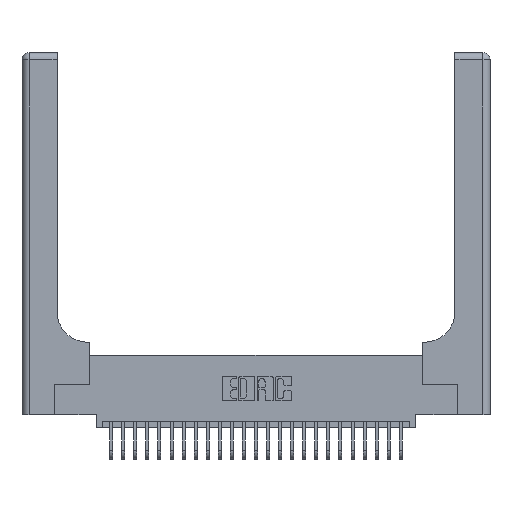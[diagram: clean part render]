
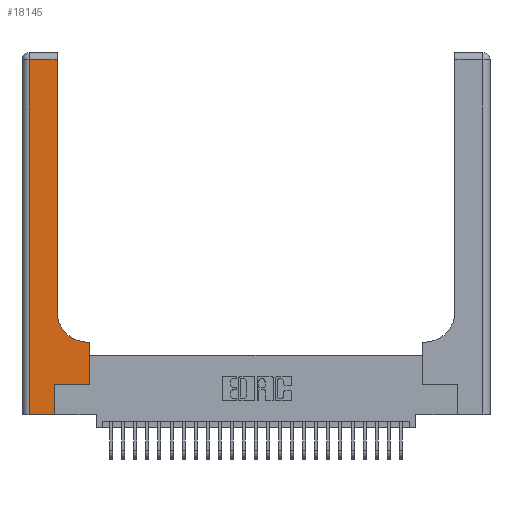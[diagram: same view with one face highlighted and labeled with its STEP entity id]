
A CAD part, top view. The second image highlights one B-rep face of the part: STEP entity #18145.
In plain terms, the highlighted planar face has unit normal (0, 0, 1).
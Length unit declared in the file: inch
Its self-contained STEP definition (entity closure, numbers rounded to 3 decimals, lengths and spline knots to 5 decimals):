
#85 = DIRECTION ( 'NONE',  ( 0., 1., 0. ) ) ;
#137 = CARTESIAN_POINT ( 'NONE',  ( 0.06, 2.94, 0.37 ) ) ;
#306 = VECTOR ( 'NONE', #23178, 39.37008 ) ;
#608 = VERTEX_POINT ( 'NONE', #1869 ) ;
#842 = DIRECTION ( 'NONE',  ( 0., 1., 0. ) ) ;
#844 = LINE ( 'NONE', #2039, #5177 ) ;
#1436 = CARTESIAN_POINT ( 'NONE',  ( 0.5415, 0.6, 0.37 ) ) ;
#1693 = AXIS2_PLACEMENT_3D ( 'NONE', #10305, #2009, #16367 ) ;
#1869 = CARTESIAN_POINT ( 'NONE',  ( 0.5585, 0.6, 0.37 ) ) ;
#2009 = DIRECTION ( 'NONE',  ( 0., 0., -1. ) ) ;
#2039 = CARTESIAN_POINT ( 'NONE',  ( 0.269, 0., 0.37 ) ) ;
#2052 = CARTESIAN_POINT ( 'NONE',  ( 0.269, 0.25, 0.37 ) ) ;
#2203 = ORIENTED_EDGE ( 'NONE', *, *, #10393, .T. ) ;
#2933 = FACE_OUTER_BOUND ( 'NONE', #15928, .T. ) ;
#3456 = LINE ( 'NONE', #26335, #13091 ) ;
#3906 = VECTOR ( 'NONE', #842, 39.37008 ) ;
#4115 = LINE ( 'NONE', #8879, #14323 ) ;
#4202 = DIRECTION ( 'NONE',  ( 0., 1., 0. ) ) ;
#4873 = CARTESIAN_POINT ( 'NONE',  ( 0.5415, 0.85, 0.37 ) ) ;
#5177 = VECTOR ( 'NONE', #4202, 39.37008 ) ;
#5640 = ORIENTED_EDGE ( 'NONE', *, *, #8423, .T. ) ;
#6949 = DIRECTION ( 'NONE',  ( 1., 0., 0. ) ) ;
#7338 = CARTESIAN_POINT ( 'NONE',  ( 0.5585, 0.25, 0.37 ) ) ;
#8005 = VERTEX_POINT ( 'NONE', #137 ) ;
#8423 = EDGE_CURVE ( 'NONE', #20503, #8005, #10038, .T. ) ;
#8587 = VERTEX_POINT ( 'NONE', #2052 ) ;
#8678 = CARTESIAN_POINT ( 'NONE',  ( 0.06, 0., 0.37 ) ) ;
#8879 = CARTESIAN_POINT ( 'NONE',  ( 0., 0., 0.37 ) ) ;
#9204 = VECTOR ( 'NONE', #85, 39.37008 ) ;
#9416 = EDGE_CURVE ( 'NONE', #608, #17862, #21445, .T. ) ;
#9902 = CARTESIAN_POINT ( 'NONE',  ( 0., 2.94, 0.37 ) ) ;
#10038 = LINE ( 'NONE', #9902, #10687 ) ;
#10199 = DIRECTION ( 'NONE',  ( 1., 0., 0. ) ) ;
#10305 = CARTESIAN_POINT ( 'NONE',  ( 0., 3., 0.37 ) ) ;
#10393 = EDGE_CURVE ( 'NONE', #22905, #20503, #25537, .T. ) ;
#10687 = VECTOR ( 'NONE', #21872, 39.37008 ) ;
#11101 = CARTESIAN_POINT ( 'NONE',  ( 0.2915, 0.6, 0.37 ) ) ;
#12141 = DIRECTION ( 'NONE',  ( 0., -1., 0. ) ) ;
#12215 = AXIS2_PLACEMENT_3D ( 'NONE', #4873, #19083, #6949 ) ;
#12929 = DIRECTION ( 'NONE',  ( 1., 0., 0. ) ) ;
#13087 = EDGE_CURVE ( 'NONE', #8587, #14572, #3456, .T. ) ;
#13091 = VECTOR ( 'NONE', #10199, 39.37008 ) ;
#13144 = VERTEX_POINT ( 'NONE', #8678 ) ;
#14158 = CARTESIAN_POINT ( 'NONE',  ( 0.06, 3., 0.37 ) ) ;
#14323 = VECTOR ( 'NONE', #12929, 39.37008 ) ;
#14556 = ORIENTED_EDGE ( 'NONE', *, *, #25193, .T. ) ;
#14564 = LINE ( 'NONE', #24639, #9204 ) ;
#14572 = VERTEX_POINT ( 'NONE', #7338 ) ;
#14680 = LINE ( 'NONE', #14158, #26073 ) ;
#15810 = ORIENTED_EDGE ( 'NONE', *, *, #26528, .T. ) ;
#15919 = ORIENTED_EDGE ( 'NONE', *, *, #24667, .T. ) ;
#15928 = EDGE_LOOP ( 'NONE', ( #2203, #5640, #14556, #15810, #15919, #17731, #22140, #22710, #20123 ) ) ;
#16367 = DIRECTION ( 'NONE',  ( -1., 0., 0. ) ) ;
#17037 = VERTEX_POINT ( 'NONE', #25013 ) ;
#17731 = ORIENTED_EDGE ( 'NONE', *, *, #13087, .T. ) ;
#17862 = VERTEX_POINT ( 'NONE', #1436 ) ;
#18099 = CARTESIAN_POINT ( 'NONE',  ( 0.2915, 0.85, 0.37 ) ) ;
#18145 = ADVANCED_FACE ( 'NONE', ( #2933 ), #18313, .F. ) ;
#18313 = PLANE ( 'NONE',  #1693 ) ;
#19083 = DIRECTION ( 'NONE',  ( 0., 0., -1. ) ) ;
#20123 = ORIENTED_EDGE ( 'NONE', *, *, #24287, .T. ) ;
#20503 = VERTEX_POINT ( 'NONE', #26325 ) ;
#21445 = LINE ( 'NONE', #11101, #306 ) ;
#21709 = EDGE_CURVE ( 'NONE', #14572, #608, #14564, .T. ) ;
#21872 = DIRECTION ( 'NONE',  ( -1., 0., 0. ) ) ;
#22140 = ORIENTED_EDGE ( 'NONE', *, *, #21709, .T. ) ;
#22710 = ORIENTED_EDGE ( 'NONE', *, *, #9416, .T. ) ;
#22905 = VERTEX_POINT ( 'NONE', #18099 ) ;
#22958 = CIRCLE ( 'NONE', #12215, 0.25 ) ;
#23178 = DIRECTION ( 'NONE',  ( -1., 0., 0. ) ) ;
#23305 = CARTESIAN_POINT ( 'NONE',  ( 0.2915, 3., 0.37 ) ) ;
#24287 = EDGE_CURVE ( 'NONE', #17862, #22905, #22958, .T. ) ;
#24639 = CARTESIAN_POINT ( 'NONE',  ( 0.5585, 0.25, 0.37 ) ) ;
#24667 = EDGE_CURVE ( 'NONE', #17037, #8587, #844, .T. ) ;
#25013 = CARTESIAN_POINT ( 'NONE',  ( 0.269, 0., 0.37 ) ) ;
#25193 = EDGE_CURVE ( 'NONE', #8005, #13144, #14680, .T. ) ;
#25537 = LINE ( 'NONE', #23305, #3906 ) ;
#26073 = VECTOR ( 'NONE', #12141, 39.37008 ) ;
#26325 = CARTESIAN_POINT ( 'NONE',  ( 0.2915, 2.94, 0.37 ) ) ;
#26335 = CARTESIAN_POINT ( 'NONE',  ( 0.269, 0.25, 0.37 ) ) ;
#26528 = EDGE_CURVE ( 'NONE', #13144, #17037, #4115, .T. ) ;
